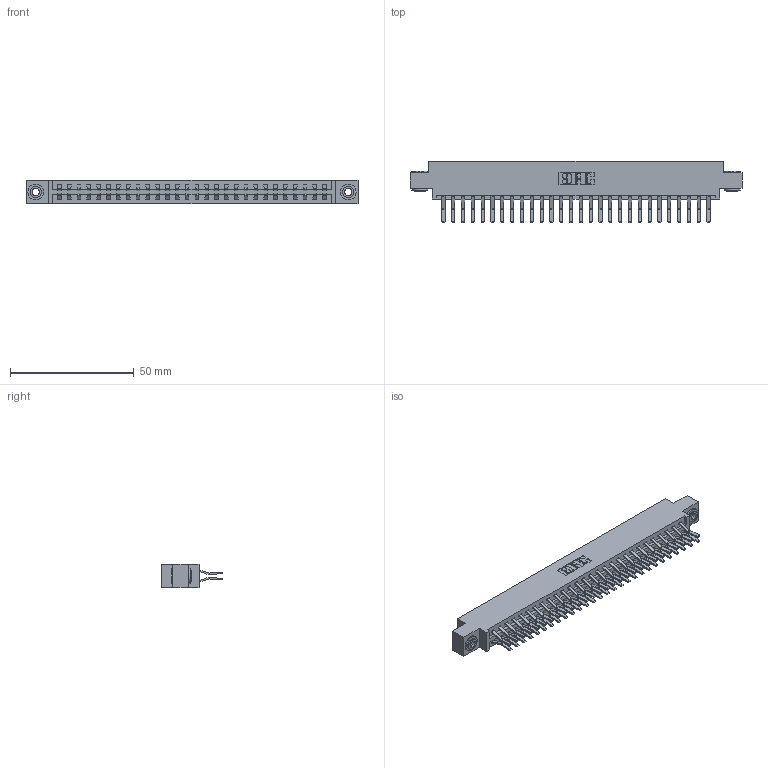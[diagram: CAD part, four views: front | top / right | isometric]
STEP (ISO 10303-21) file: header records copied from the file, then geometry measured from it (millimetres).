
FILE_DESCRIPTION (( 'STEP AP203' ), '1' );
FILE_NAME ('387-056-560-803.STEP', '2019-10-19T08:11:41', ( '' ), ( '' ), 'SwSTEP 2.0', 'SolidWorks 2016', '' );
FILE_SCHEMA (( 'CONFIG_CONTROL_DESIGN' ));
Length unit declared in the file: inch
Products named in the file (4): 387-056-560-803; 345-292-001_560 Tail; 337 Part_0.170 Offset - 0.156 Dia-TH; 345-250-002_345-250-002-102
Assembly tree (59 placements, depth 2):
  387-056-560-803
    337 Part_0.170 Offset - 0.156 Dia-TH
    345-292-001_560 Tail  x56
    345-250-002_345-250-002-102  x2
Bounding box: 133.96 x 24.78 x 9.4 mm (x, y, z)
Volume: 14200.3 mm3; surface area: 17312.1 mm2
Topology: 59 solids, 59 shells, 3292 faces, 9751 edges, 6422 vertices
Faces by surface type: plane 2212, cylinder 1072, cone 8
Entity records: 24390 total; most frequent: CARTESIAN_POINT 4097, ORIENTED_EDGE 4026, DIRECTION 3547, EDGE_CURVE 2013, VECTOR 1857, LINE 1857, VERTEX_POINT 1338, AXIS2_PLACEMENT_3D 845
